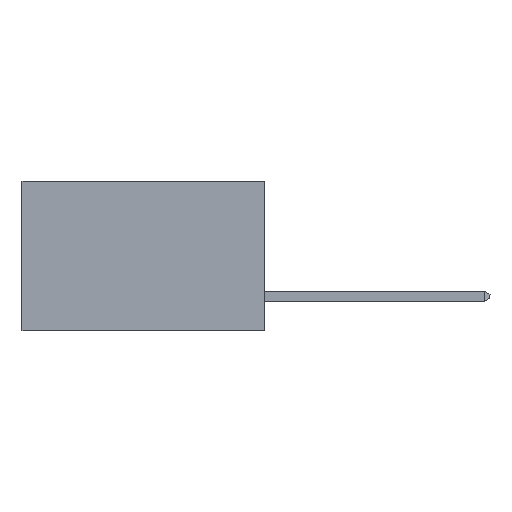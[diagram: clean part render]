
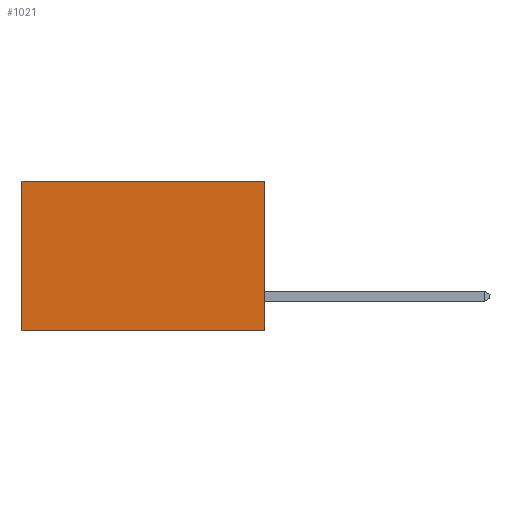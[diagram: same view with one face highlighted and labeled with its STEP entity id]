
A CAD part, left-side view. The second image highlights one B-rep face of the part: STEP entity #1021.
In plain terms, the highlighted planar face has unit normal (-1, 0, 0).
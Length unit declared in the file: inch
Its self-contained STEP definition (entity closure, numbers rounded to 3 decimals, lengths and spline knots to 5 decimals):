
#72 = EDGE_CURVE ( 'NONE', #7140, #9566, #7773, .T. ) ;
#127 = CARTESIAN_POINT ( 'NONE',  ( 0.2615, 0., -0.37 ) ) ;
#159 = AXIS2_PLACEMENT_3D ( 'NONE', #127, #2427, #4030 ) ;
#369 = CARTESIAN_POINT ( 'NONE',  ( 0.2615, 0.6, -0.37 ) ) ;
#435 = CARTESIAN_POINT ( 'NONE',  ( 0.2615, 0.6, 0. ) ) ;
#844 = CARTESIAN_POINT ( 'NONE',  ( 0.2615, 0., -0.37 ) ) ;
#883 = FACE_OUTER_BOUND ( 'NONE', #2067, .T. ) ;
#985 = PLANE ( 'NONE',  #159 ) ;
#1021 = ADVANCED_FACE ( 'NONE', ( #883 ), #985, .F. ) ;
#1176 = DIRECTION ( 'NONE',  ( 0., 1., 0. ) ) ;
#1634 = VECTOR ( 'NONE', #4857, 39.37008 ) ;
#1643 = DIRECTION ( 'NONE',  ( 0., 1., 0. ) ) ;
#1859 = LINE ( 'NONE', #369, #1634 ) ;
#2067 = EDGE_LOOP ( 'NONE', ( #9123, #4795, #6245, #9602 ) ) ;
#2427 = DIRECTION ( 'NONE',  ( 1., 0., 0. ) ) ;
#3090 = EDGE_CURVE ( 'NONE', #9566, #4176, #1859, .T. ) ;
#3919 = CARTESIAN_POINT ( 'NONE',  ( 0.2615, 0.6, -0.37 ) ) ;
#4030 = DIRECTION ( 'NONE',  ( 0., 0., -1. ) ) ;
#4176 = VERTEX_POINT ( 'NONE', #3919 ) ;
#4404 = CARTESIAN_POINT ( 'NONE',  ( 0.2615, 0., 0. ) ) ;
#4795 = ORIENTED_EDGE ( 'NONE', *, *, #8500, .F. ) ;
#4857 = DIRECTION ( 'NONE',  ( 0., 0., -1. ) ) ;
#5221 = LINE ( 'NONE', #7602, #8485 ) ;
#5275 = DIRECTION ( 'NONE',  ( 0., 0., -1. ) ) ;
#6245 = ORIENTED_EDGE ( 'NONE', *, *, #6790, .F. ) ;
#6749 = VERTEX_POINT ( 'NONE', #6828 ) ;
#6790 = EDGE_CURVE ( 'NONE', #7140, #6749, #5221, .T. ) ;
#6828 = CARTESIAN_POINT ( 'NONE',  ( 0.2615, 0., -0.37 ) ) ;
#7001 = CARTESIAN_POINT ( 'NONE',  ( 0.2615, 0., 0. ) ) ;
#7140 = VERTEX_POINT ( 'NONE', #4404 ) ;
#7216 = VECTOR ( 'NONE', #1176, 39.37008 ) ;
#7602 = CARTESIAN_POINT ( 'NONE',  ( 0.2615, 0., -0.37 ) ) ;
#7773 = LINE ( 'NONE', #7001, #7216 ) ;
#7960 = LINE ( 'NONE', #844, #9307 ) ;
#8485 = VECTOR ( 'NONE', #5275, 39.37008 ) ;
#8500 = EDGE_CURVE ( 'NONE', #6749, #4176, #7960, .T. ) ;
#9123 = ORIENTED_EDGE ( 'NONE', *, *, #3090, .T. ) ;
#9307 = VECTOR ( 'NONE', #1643, 39.37008 ) ;
#9566 = VERTEX_POINT ( 'NONE', #435 ) ;
#9602 = ORIENTED_EDGE ( 'NONE', *, *, #72, .T. ) ;
